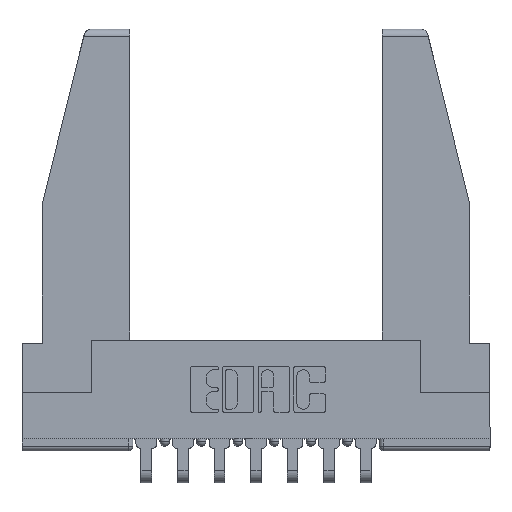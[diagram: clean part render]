
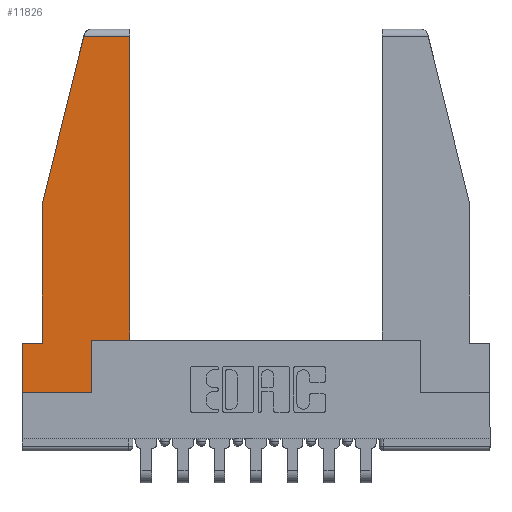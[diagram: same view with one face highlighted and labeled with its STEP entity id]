
A CAD part, top view. The second image highlights one B-rep face of the part: STEP entity #11826.
In plain terms, the highlighted planar face has unit normal (0, 0, 1).
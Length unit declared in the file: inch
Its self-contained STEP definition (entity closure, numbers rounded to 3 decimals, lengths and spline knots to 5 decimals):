
#209 = CARTESIAN_POINT ( 'NONE',  ( 0., 1.52, 0. ) ) ;
#424 = EDGE_CURVE ( 'NONE', #7100, #1929, #4271, .T. ) ;
#447 = AXIS2_PLACEMENT_3D ( 'NONE', #4826, #4921, #1856 ) ;
#575 = EDGE_CURVE ( 'NONE', #5219, #7100, #10489, .T. ) ;
#589 = VECTOR ( 'NONE', #3433, 39.37008 ) ;
#1384 = LINE ( 'NONE', #5724, #1991 ) ;
#1562 = ORIENTED_EDGE ( 'NONE', *, *, #5215, .T. ) ;
#1856 = DIRECTION ( 'NONE',  ( 1., 0., 0. ) ) ;
#1918 = EDGE_CURVE ( 'NONE', #12000, #10217, #8701, .T. ) ;
#1929 = VERTEX_POINT ( 'NONE', #8553 ) ;
#1991 = VECTOR ( 'NONE', #10580, 39.37008 ) ;
#2033 = VECTOR ( 'NONE', #4797, 39.37008 ) ;
#2080 = ORIENTED_EDGE ( 'NONE', *, *, #7768, .T. ) ;
#2231 = ORIENTED_EDGE ( 'NONE', *, *, #424, .T. ) ;
#2300 = VERTEX_POINT ( 'NONE', #10335 ) ;
#2463 = VECTOR ( 'NONE', #3326, 39.37008 ) ;
#2552 = CARTESIAN_POINT ( 'NONE',  ( 0., 0.21, 0. ) ) ;
#2795 = DIRECTION ( 'NONE',  ( -1., 0., 0. ) ) ;
#2804 = LINE ( 'NONE', #10716, #2033 ) ;
#2915 = PLANE ( 'NONE',  #447 ) ;
#2953 = LINE ( 'NONE', #10250, #10590 ) ;
#3130 = ORIENTED_EDGE ( 'NONE', *, *, #8222, .T. ) ;
#3326 = DIRECTION ( 'NONE',  ( 0., -1., 0. ) ) ;
#3433 = DIRECTION ( 'NONE',  ( -0.239, -0.971, 0. ) ) ;
#3560 = LINE ( 'NONE', #209, #7012 ) ;
#4087 = VERTEX_POINT ( 'NONE', #9763 ) ;
#4108 = VECTOR ( 'NONE', #2795, 39.37008 ) ;
#4271 = LINE ( 'NONE', #10477, #8643 ) ;
#4274 = DIRECTION ( 'NONE',  ( 0., 1., 0. ) ) ;
#4416 = CARTESIAN_POINT ( 'NONE',  ( 0.086, 0.8, 0. ) ) ;
#4481 = EDGE_LOOP ( 'NONE', ( #2080, #6187, #8996, #9824, #7812, #2231, #1562, #3130, #12824 ) ) ;
#4797 = DIRECTION ( 'NONE',  ( 1., 0., 0. ) ) ;
#4826 = CARTESIAN_POINT ( 'NONE',  ( 0., 0., 0. ) ) ;
#4893 = CARTESIAN_POINT ( 'NONE',  ( 0.297, 0.223, 0. ) ) ;
#4921 = DIRECTION ( 'NONE',  ( 0., 0., 1. ) ) ;
#5215 = EDGE_CURVE ( 'NONE', #1929, #8768, #2804, .T. ) ;
#5219 = VERTEX_POINT ( 'NONE', #5728 ) ;
#5380 = VERTEX_POINT ( 'NONE', #11997 ) ;
#5406 = CARTESIAN_POINT ( 'NONE',  ( 0.271, 1.55, 0. ) ) ;
#5724 = CARTESIAN_POINT ( 'NONE',  ( 0.461, 0.223, 0. ) ) ;
#5728 = CARTESIAN_POINT ( 'NONE',  ( 0.086, 0.21, 0. ) ) ;
#6187 = ORIENTED_EDGE ( 'NONE', *, *, #8740, .T. ) ;
#6228 = CARTESIAN_POINT ( 'NONE',  ( 0.086, 0.8, 0. ) ) ;
#6261 = DIRECTION ( 'NONE',  ( -1., 0., 0. ) ) ;
#6760 = FACE_OUTER_BOUND ( 'NONE', #4481, .T. ) ;
#7012 = VECTOR ( 'NONE', #6261, 39.37008 ) ;
#7100 = VERTEX_POINT ( 'NONE', #2552 ) ;
#7571 = VECTOR ( 'NONE', #8950, 39.37008 ) ;
#7768 = EDGE_CURVE ( 'NONE', #4087, #2300, #1384, .T. ) ;
#7812 = ORIENTED_EDGE ( 'NONE', *, *, #575, .T. ) ;
#8222 = EDGE_CURVE ( 'NONE', #8768, #5380, #2953, .T. ) ;
#8332 = CARTESIAN_POINT ( 'NONE',  ( 0.297, 0., 0. ) ) ;
#8553 = CARTESIAN_POINT ( 'NONE',  ( 0., 0., 0. ) ) ;
#8619 = DIRECTION ( 'NONE',  ( 0., -1., 0. ) ) ;
#8643 = VECTOR ( 'NONE', #8619, 39.37008 ) ;
#8701 = LINE ( 'NONE', #5406, #589 ) ;
#8705 = CARTESIAN_POINT ( 'NONE',  ( 0., 0.21, 0. ) ) ;
#8740 = EDGE_CURVE ( 'NONE', #2300, #12000, #3560, .T. ) ;
#8768 = VERTEX_POINT ( 'NONE', #8332 ) ;
#8950 = DIRECTION ( 'NONE',  ( 1., 0., 0. ) ) ;
#8996 = ORIENTED_EDGE ( 'NONE', *, *, #1918, .T. ) ;
#9763 = CARTESIAN_POINT ( 'NONE',  ( 0.461, 0.223, 0. ) ) ;
#9776 = EDGE_CURVE ( 'NONE', #10217, #5219, #12097, .T. ) ;
#9824 = ORIENTED_EDGE ( 'NONE', *, *, #9776, .T. ) ;
#10217 = VERTEX_POINT ( 'NONE', #6228 ) ;
#10250 = CARTESIAN_POINT ( 'NONE',  ( 0.297, 0., 0. ) ) ;
#10284 = CARTESIAN_POINT ( 'NONE',  ( 0.2636, 1.52, 0. ) ) ;
#10335 = CARTESIAN_POINT ( 'NONE',  ( 0.461, 1.52, 0. ) ) ;
#10477 = CARTESIAN_POINT ( 'NONE',  ( 0., 0.21, 0. ) ) ;
#10489 = LINE ( 'NONE', #8705, #4108 ) ;
#10510 = LINE ( 'NONE', #4893, #7571 ) ;
#10580 = DIRECTION ( 'NONE',  ( 0., 1., 0. ) ) ;
#10590 = VECTOR ( 'NONE', #4274, 39.37008 ) ;
#10716 = CARTESIAN_POINT ( 'NONE',  ( 0., 0., 0. ) ) ;
#11336 = EDGE_CURVE ( 'NONE', #5380, #4087, #10510, .T. ) ;
#11826 = ADVANCED_FACE ( 'NONE', ( #6760 ), #2915, .T. ) ;
#11997 = CARTESIAN_POINT ( 'NONE',  ( 0.297, 0.223, 0. ) ) ;
#12000 = VERTEX_POINT ( 'NONE', #10284 ) ;
#12097 = LINE ( 'NONE', #4416, #2463 ) ;
#12824 = ORIENTED_EDGE ( 'NONE', *, *, #11336, .T. ) ;
